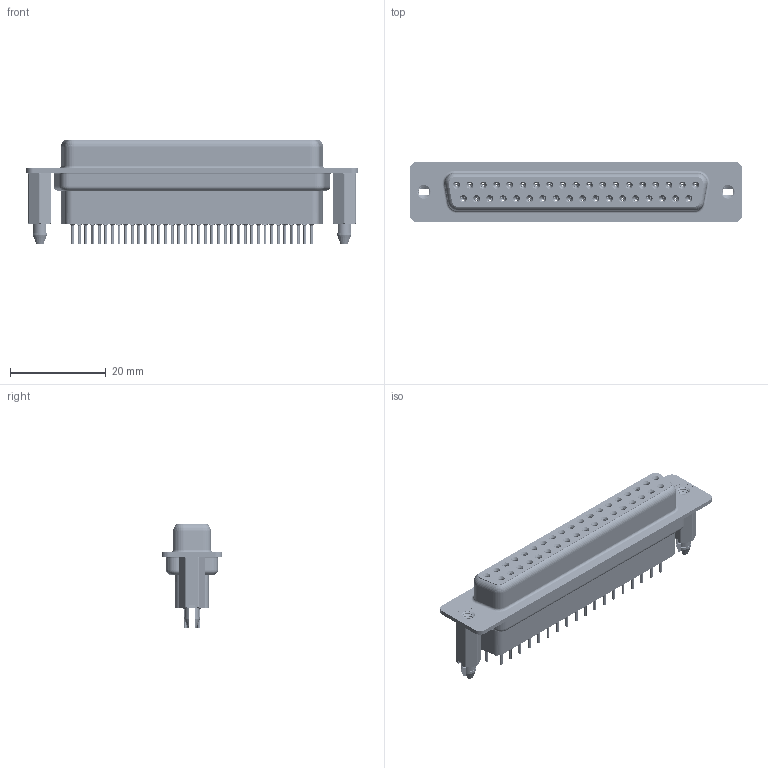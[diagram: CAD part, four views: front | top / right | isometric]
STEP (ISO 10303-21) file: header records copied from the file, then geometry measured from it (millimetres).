
FILE_DESCRIPTION (( 'STEP AP203' ), '1' );
FILE_NAME ('628-037-221-076.STEP', '2020-07-14T17:00:39', ( '' ), ( '' ), 'SwSTEP 2.0', 'SolidWorks 2020', '' );
FILE_SCHEMA (( 'CONFIG_CONTROL_DESIGN' ));
Length unit declared in the file: millimetre
Products named in the file (7): 628-037-221-076; 628 Contact Row 1_21H; 628 4-40 Threaded Boardlock_HP; 628 Housing_37 HP; 628 Shell Rear_37 Contacts; 628 Shell Front_37 Contacts; 628 Contact Row 2_21H
Assembly tree (42 placements, depth 2):
  628-037-221-076
    628 Housing_37 HP
    628 Shell Front_37 Contacts
    628 Shell Rear_37 Contacts
    628 Contact Row 1_21H  x19
    628 Contact Row 2_21H  x18
    628 4-40 Threaded Boardlock_HP  x2
Bounding box: 69.3 x 12.6 x 21.9 mm (x, y, z)
Volume: 7283.5 mm3; surface area: 16649.2 mm2
Topology: 42 solids, 42 shells, 4944 faces, 12729 edges, 7952 vertices
Faces by surface type: cylinder 1426, plane 1246, torus 951, bspline 750, cone 571
Entity records: 36272 total; most frequent: CARTESIAN_POINT 10897, DIRECTION 5218, ORIENTED_EDGE 4780, EDGE_CURVE 2390, AXIS2_PLACEMENT_3D 2181, VERTEX_POINT 1517, EDGE_LOOP 1211, CIRCLE 1177
